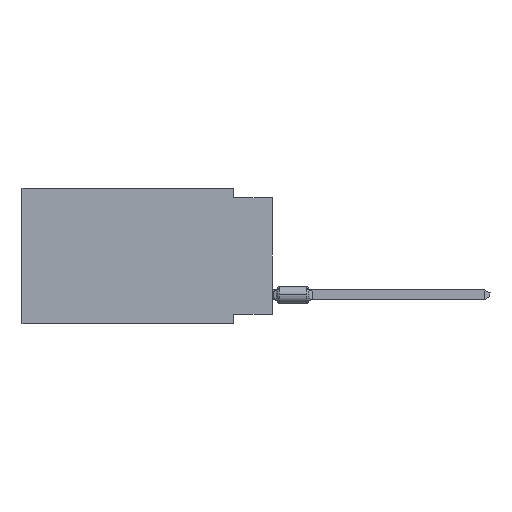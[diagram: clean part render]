
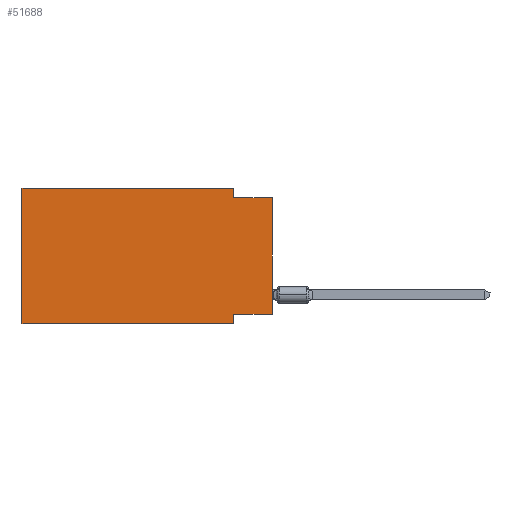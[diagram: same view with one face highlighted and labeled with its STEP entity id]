
A CAD part, left-side view. The second image highlights one B-rep face of the part: STEP entity #51688.
In plain terms, the highlighted planar face has unit normal (-1, 0, 0).
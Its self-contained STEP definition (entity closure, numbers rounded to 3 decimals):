
#1438 = DIRECTION ( 'NONE',  ( 0., 0., -1. ) ) ;
#6748 = DIRECTION ( 'NONE',  ( 0., 0., 1. ) ) ;
#8239 = CARTESIAN_POINT ( 'NONE',  ( 0., 0., 0. ) ) ;
#8718 = CARTESIAN_POINT ( 'NONE',  ( 0., 2.54, -8.89 ) ) ;
#9156 = ORIENTED_EDGE ( 'NONE', *, *, #63734, .F. ) ;
#10224 = CARTESIAN_POINT ( 'NONE',  ( 0., 2.54, -0.635 ) ) ;
#11342 = EDGE_CURVE ( 'NONE', #51685, #89510, #92931, .T. ) ;
#16167 = EDGE_CURVE ( 'NONE', #65120, #89510, #34316, .T. ) ;
#16303 = DIRECTION ( 'NONE',  ( 1., 0., 0. ) ) ;
#17171 = DIRECTION ( 'NONE',  ( 0., 0., 1. ) ) ;
#17238 = DIRECTION ( 'NONE',  ( 0., 1., 0. ) ) ;
#21952 = VERTEX_POINT ( 'NONE', #60672 ) ;
#23939 = ORIENTED_EDGE ( 'NONE', *, *, #33182, .F. ) ;
#24805 = LINE ( 'NONE', #85776, #49049 ) ;
#25344 = ORIENTED_EDGE ( 'NONE', *, *, #11342, .T. ) ;
#25612 = CARTESIAN_POINT ( 'NONE',  ( 0., 16.383, 0. ) ) ;
#28242 = VERTEX_POINT ( 'NONE', #88022 ) ;
#30204 = CARTESIAN_POINT ( 'NONE',  ( 0., 2.54, 0. ) ) ;
#31921 = PLANE ( 'NONE',  #81138 ) ;
#33182 = EDGE_CURVE ( 'NONE', #28242, #65120, #24805, .T. ) ;
#34316 = LINE ( 'NONE', #80672, #71724 ) ;
#35551 = ORIENTED_EDGE ( 'NONE', *, *, #71081, .F. ) ;
#40829 = CARTESIAN_POINT ( 'NONE',  ( 0., 16.383, 0. ) ) ;
#41318 = DIRECTION ( 'NONE',  ( 0., -1., 0. ) ) ;
#46350 = VERTEX_POINT ( 'NONE', #25612 ) ;
#47572 = DIRECTION ( 'NONE',  ( 0., -1., 0. ) ) ;
#48439 = VECTOR ( 'NONE', #47572, 1000. ) ;
#48760 = CARTESIAN_POINT ( 'NONE',  ( 0., 16.383, 0. ) ) ;
#49049 = VECTOR ( 'NONE', #17238, 1000. ) ;
#50419 = VERTEX_POINT ( 'NONE', #83399 ) ;
#51668 = EDGE_CURVE ( 'NONE', #28242, #21952, #69203, .T. ) ;
#51685 = VERTEX_POINT ( 'NONE', #69696 ) ;
#51688 = ADVANCED_FACE ( 'NONE', ( #70190 ), #31921, .F. ) ;
#52783 = ORIENTED_EDGE ( 'NONE', *, *, #94112, .F. ) ;
#53388 = DIRECTION ( 'NONE',  ( 0., 0., -1. ) ) ;
#56455 = VECTOR ( 'NONE', #41318, 1000. ) ;
#56669 = CARTESIAN_POINT ( 'NONE',  ( 0., 2.54, -8.255 ) ) ;
#57438 = LINE ( 'NONE', #87679, #56455 ) ;
#60460 = VECTOR ( 'NONE', #17171, 1000. ) ;
#60672 = CARTESIAN_POINT ( 'NONE',  ( 0., 0., -0.635 ) ) ;
#62404 = VECTOR ( 'NONE', #64369, 1000. ) ;
#62650 = ORIENTED_EDGE ( 'NONE', *, *, #16167, .F. ) ;
#63734 = EDGE_CURVE ( 'NONE', #51685, #46350, #77634, .T. ) ;
#64369 = DIRECTION ( 'NONE',  ( 0., -1., 0. ) ) ;
#65120 = VERTEX_POINT ( 'NONE', #56669 ) ;
#65853 = LINE ( 'NONE', #48760, #62404 ) ;
#67172 = VERTEX_POINT ( 'NONE', #10224 ) ;
#69203 = LINE ( 'NONE', #8239, #77976 ) ;
#69696 = CARTESIAN_POINT ( 'NONE',  ( 0., 16.383, -8.89 ) ) ;
#70190 = FACE_OUTER_BOUND ( 'NONE', #73734, .T. ) ;
#71078 = VECTOR ( 'NONE', #53388, 1000. ) ;
#71081 = EDGE_CURVE ( 'NONE', #67172, #21952, #57438, .T. ) ;
#71724 = VECTOR ( 'NONE', #1438, 1000. ) ;
#73734 = EDGE_LOOP ( 'NONE', ( #89094, #35551, #76871, #52783, #9156, #25344, #62650, #23939 ) ) ;
#76871 = ORIENTED_EDGE ( 'NONE', *, *, #83433, .F. ) ;
#77634 = LINE ( 'NONE', #40829, #60460 ) ;
#77976 = VECTOR ( 'NONE', #6748, 1000. ) ;
#80672 = CARTESIAN_POINT ( 'NONE',  ( 0., 2.54, -8.89 ) ) ;
#81138 = AXIS2_PLACEMENT_3D ( 'NONE', #85333, #16303, #93385 ) ;
#83110 = LINE ( 'NONE', #30204, #71078 ) ;
#83399 = CARTESIAN_POINT ( 'NONE',  ( 0., 2.54, 0. ) ) ;
#83433 = EDGE_CURVE ( 'NONE', #50419, #67172, #83110, .T. ) ;
#85333 = CARTESIAN_POINT ( 'NONE',  ( 0., 16.383, 0. ) ) ;
#85776 = CARTESIAN_POINT ( 'NONE',  ( 0., 0., -8.255 ) ) ;
#85868 = CARTESIAN_POINT ( 'NONE',  ( 0., 16.383, -8.89 ) ) ;
#87679 = CARTESIAN_POINT ( 'NONE',  ( 0., 0., -0.635 ) ) ;
#88022 = CARTESIAN_POINT ( 'NONE',  ( 0., 0., -8.255 ) ) ;
#89094 = ORIENTED_EDGE ( 'NONE', *, *, #51668, .T. ) ;
#89510 = VERTEX_POINT ( 'NONE', #8718 ) ;
#92931 = LINE ( 'NONE', #85868, #48439 ) ;
#93385 = DIRECTION ( 'NONE',  ( 0., 0., -1. ) ) ;
#94112 = EDGE_CURVE ( 'NONE', #46350, #50419, #65853, .T. ) ;
